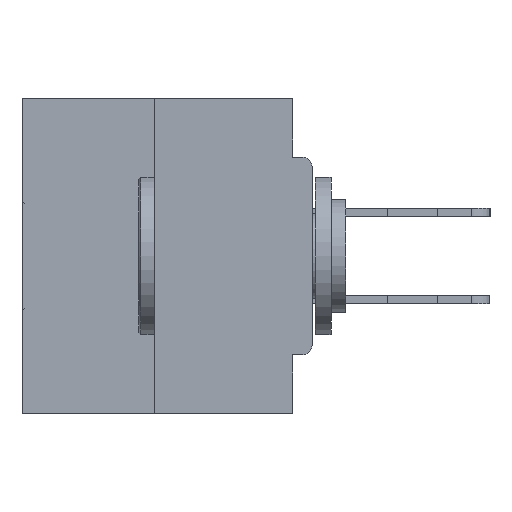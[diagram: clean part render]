
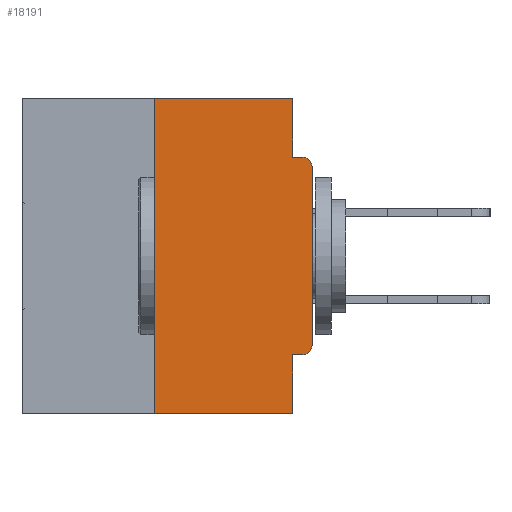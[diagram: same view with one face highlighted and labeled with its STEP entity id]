
A CAD part, left-side view. The second image highlights one B-rep face of the part: STEP entity #18191.
In plain terms, the highlighted planar face has unit normal (-1, 0, 0).
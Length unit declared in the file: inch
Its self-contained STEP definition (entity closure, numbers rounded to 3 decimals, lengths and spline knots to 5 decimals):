
#103 = DIRECTION ( 'NONE',  ( 0., 0., 1. ) ) ;
#228 = EDGE_CURVE ( 'NONE', #24305, #41246, #36857, .T. ) ;
#1974 = DIRECTION ( 'NONE',  ( 0., 0., -1. ) ) ;
#4390 = VERTEX_POINT ( 'NONE', #13432 ) ;
#4446 = DIRECTION ( 'NONE',  ( -1., 0., 0. ) ) ;
#5122 = CARTESIAN_POINT ( 'NONE',  ( 0., 0.015, -0.3915 ) ) ;
#5417 = ORIENTED_EDGE ( 'NONE', *, *, #39782, .T. ) ;
#5439 = ORIENTED_EDGE ( 'NONE', *, *, #29354, .T. ) ;
#6371 = ORIENTED_EDGE ( 'NONE', *, *, #25447, .T. ) ;
#6886 = CARTESIAN_POINT ( 'NONE',  ( 0., 0.46, 0. ) ) ;
#7464 = VERTEX_POINT ( 'NONE', #34262 ) ;
#7972 = VECTOR ( 'NONE', #12692, 39.37008 ) ;
#8145 = VERTEX_POINT ( 'NONE', #10415 ) ;
#8596 = LINE ( 'NONE', #16424, #39526 ) ;
#9970 = AXIS2_PLACEMENT_3D ( 'NONE', #12853, #22806, #31863 ) ;
#9973 = CARTESIAN_POINT ( 'NONE',  ( 0., 0.015, -0.0935 ) ) ;
#9983 = VERTEX_POINT ( 'NONE', #22271 ) ;
#10415 = CARTESIAN_POINT ( 'NONE',  ( 0., 0.031, -0.5 ) ) ;
#11400 = LINE ( 'NONE', #16168, #20725 ) ;
#11575 = CARTESIAN_POINT ( 'NONE',  ( 0., 0.015, -0.1085 ) ) ;
#11949 = AXIS2_PLACEMENT_3D ( 'NONE', #5122, #21765, #1974 ) ;
#12233 = VERTEX_POINT ( 'NONE', #42303 ) ;
#12345 = EDGE_CURVE ( 'NONE', #40365, #4390, #17448, .T. ) ;
#12692 = DIRECTION ( 'NONE',  ( 0., -1., 0. ) ) ;
#12853 = CARTESIAN_POINT ( 'NONE',  ( 0., 0.46, 0. ) ) ;
#13432 = CARTESIAN_POINT ( 'NONE',  ( 0., 0.25, 0. ) ) ;
#13542 = CARTESIAN_POINT ( 'NONE',  ( 0., 0.46, -0.5 ) ) ;
#13923 = CARTESIAN_POINT ( 'NONE',  ( 0., 0., -0.4065 ) ) ;
#14690 = VECTOR ( 'NONE', #30124, 39.37008 ) ;
#16168 = CARTESIAN_POINT ( 'NONE',  ( 0., 0.031, -0.5 ) ) ;
#16290 = ORIENTED_EDGE ( 'NONE', *, *, #19038, .F. ) ;
#16424 = CARTESIAN_POINT ( 'NONE',  ( 0., 0., 0. ) ) ;
#17105 = CIRCLE ( 'NONE', #33255, 0.015 ) ;
#17379 = DIRECTION ( 'NONE',  ( 0., 1., 0. ) ) ;
#17448 = LINE ( 'NONE', #22542, #18996 ) ;
#18191 = ADVANCED_FACE ( 'NONE', ( #31576 ), #34774, .F. ) ;
#18275 = EDGE_CURVE ( 'NONE', #7464, #24305, #38290, .T. ) ;
#18996 = VECTOR ( 'NONE', #32322, 39.37008 ) ;
#19038 = EDGE_CURVE ( 'NONE', #9983, #12233, #19647, .T. ) ;
#19647 = LINE ( 'NONE', #13923, #40745 ) ;
#20725 = VECTOR ( 'NONE', #22655, 39.37008 ) ;
#20928 = EDGE_LOOP ( 'NONE', ( #34817, #28443, #5439, #30908, #16290, #5417, #6371, #32727, #23949, #33277 ) ) ;
#21765 = DIRECTION ( 'NONE',  ( -1., 0., 0. ) ) ;
#21947 = EDGE_CURVE ( 'NONE', #37986, #41246, #17105, .T. ) ;
#22069 = LINE ( 'NONE', #13542, #38545 ) ;
#22252 = EDGE_CURVE ( 'NONE', #12233, #8145, #11400, .T. ) ;
#22271 = CARTESIAN_POINT ( 'NONE',  ( 0., 0.015, -0.4065 ) ) ;
#22542 = CARTESIAN_POINT ( 'NONE',  ( 0., 0.25, 0. ) ) ;
#22655 = DIRECTION ( 'NONE',  ( 0., 0., -1. ) ) ;
#22806 = DIRECTION ( 'NONE',  ( 1., 0., 0. ) ) ;
#23255 = CARTESIAN_POINT ( 'NONE',  ( 0., 0., -0.3915 ) ) ;
#23363 = DIRECTION ( 'NONE',  ( 0., 0., -1. ) ) ;
#23949 = ORIENTED_EDGE ( 'NONE', *, *, #228, .F. ) ;
#24305 = VERTEX_POINT ( 'NONE', #30387 ) ;
#25447 = EDGE_CURVE ( 'NONE', #31756, #37986, #8596, .T. ) ;
#26458 = EDGE_CURVE ( 'NONE', #4390, #7464, #29114, .T. ) ;
#27522 = DIRECTION ( 'NONE',  ( 0., -1., 0. ) ) ;
#28443 = ORIENTED_EDGE ( 'NONE', *, *, #12345, .F. ) ;
#29114 = LINE ( 'NONE', #6886, #14690 ) ;
#29354 = EDGE_CURVE ( 'NONE', #40365, #8145, #22069, .T. ) ;
#29452 = CARTESIAN_POINT ( 'NONE',  ( 0., 0.25, -0.5 ) ) ;
#29514 = VECTOR ( 'NONE', #23363, 39.37008 ) ;
#30124 = DIRECTION ( 'NONE',  ( 0., -1., 0. ) ) ;
#30266 = CARTESIAN_POINT ( 'NONE',  ( 0., 0.031, 0. ) ) ;
#30387 = CARTESIAN_POINT ( 'NONE',  ( 0., 0.031, -0.0935 ) ) ;
#30908 = ORIENTED_EDGE ( 'NONE', *, *, #22252, .F. ) ;
#31576 = FACE_OUTER_BOUND ( 'NONE', #20928, .T. ) ;
#31756 = VERTEX_POINT ( 'NONE', #23255 ) ;
#31863 = DIRECTION ( 'NONE',  ( 0., 0., -1. ) ) ;
#32322 = DIRECTION ( 'NONE',  ( 0., 0., 1. ) ) ;
#32727 = ORIENTED_EDGE ( 'NONE', *, *, #21947, .T. ) ;
#33255 = AXIS2_PLACEMENT_3D ( 'NONE', #11575, #4446, #41260 ) ;
#33277 = ORIENTED_EDGE ( 'NONE', *, *, #18275, .F. ) ;
#33978 = CIRCLE ( 'NONE', #11949, 0.015 ) ;
#34262 = CARTESIAN_POINT ( 'NONE',  ( 0., 0.031, 0. ) ) ;
#34774 = PLANE ( 'NONE',  #9970 ) ;
#34817 = ORIENTED_EDGE ( 'NONE', *, *, #26458, .F. ) ;
#36857 = LINE ( 'NONE', #42520, #7972 ) ;
#37986 = VERTEX_POINT ( 'NONE', #38373 ) ;
#38290 = LINE ( 'NONE', #30266, #29514 ) ;
#38373 = CARTESIAN_POINT ( 'NONE',  ( 0., 0., -0.1085 ) ) ;
#38545 = VECTOR ( 'NONE', #27522, 39.37008 ) ;
#39526 = VECTOR ( 'NONE', #103, 39.37008 ) ;
#39782 = EDGE_CURVE ( 'NONE', #9983, #31756, #33978, .T. ) ;
#40365 = VERTEX_POINT ( 'NONE', #29452 ) ;
#40745 = VECTOR ( 'NONE', #17379, 39.37008 ) ;
#41246 = VERTEX_POINT ( 'NONE', #9973 ) ;
#41260 = DIRECTION ( 'NONE',  ( 0., 0., -1. ) ) ;
#42303 = CARTESIAN_POINT ( 'NONE',  ( 0., 0.031, -0.4065 ) ) ;
#42520 = CARTESIAN_POINT ( 'NONE',  ( 0., 0., -0.0935 ) ) ;
